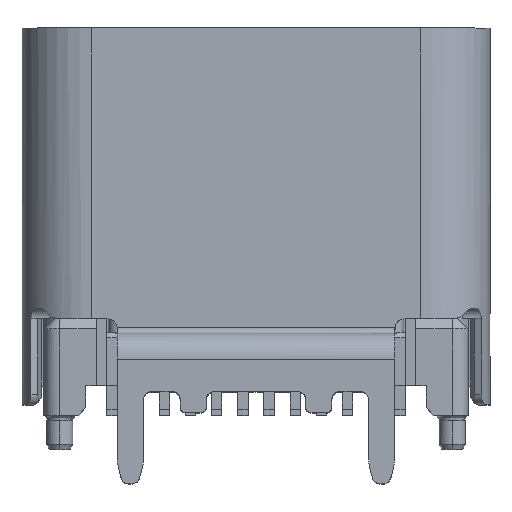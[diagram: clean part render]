
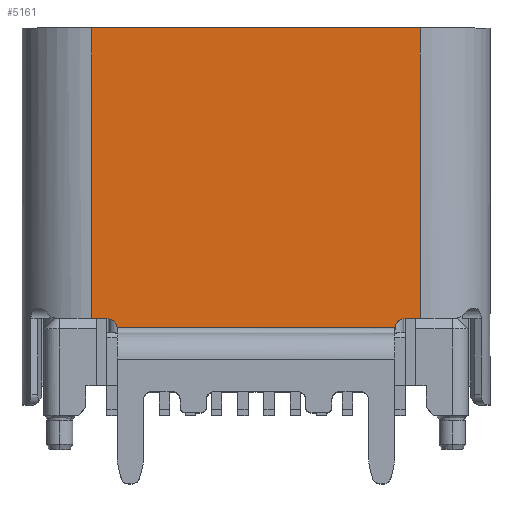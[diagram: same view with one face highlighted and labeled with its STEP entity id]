
A CAD part, top view. The second image highlights one B-rep face of the part: STEP entity #5161.
In plain terms, the highlighted face is planar.
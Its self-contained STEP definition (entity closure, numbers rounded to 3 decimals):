
#84 = EDGE_CURVE ( 'NONE', #32273, #32758, #39885, .T. ) ;
#189 = LINE ( 'NONE', #25824, #6939 ) ;
#207 = VERTEX_POINT ( 'NONE', #1972 ) ;
#1298 = DIRECTION ( 'NONE',  ( 0., 0., -1. ) ) ;
#1972 = CARTESIAN_POINT ( 'NONE',  ( 10.786, 16.807, 15.783 ) ) ;
#2573 = DIRECTION ( 'NONE',  ( 0., 0., -1. ) ) ;
#3392 = DIRECTION ( 'NONE',  ( 0., 1., 0. ) ) ;
#4640 = DIRECTION ( 'NONE',  ( -1., 0., 0. ) ) ;
#4763 = PLANE ( 'NONE',  #21060 ) ;
#5161 = ADVANCED_FACE ( 'NONE', ( #22440 ), #4763, .F. ) ;
#5346 = VECTOR ( 'NONE', #15647, 1000. ) ;
#5820 = LINE ( 'NONE', #41837, #13545 ) ;
#6440 = ORIENTED_EDGE ( 'NONE', *, *, #10337, .F. ) ;
#6939 = VECTOR ( 'NONE', #4640, 1000. ) ;
#7662 = CARTESIAN_POINT ( 'NONE',  ( 7.646, 11.257, 15.783 ) ) ;
#7954 = CARTESIAN_POINT ( 'NONE',  ( 10.786, 11.257, 15.783 ) ) ;
#8093 = LINE ( 'NONE', #14927, #35427 ) ;
#10337 = EDGE_CURVE ( 'NONE', #32758, #207, #46252, .T. ) ;
#10343 = DIRECTION ( 'NONE',  ( 1., 0., 0. ) ) ;
#10352 = CARTESIAN_POINT ( 'NONE',  ( 4.796, 17.007, 15.783 ) ) ;
#11971 = CIRCLE ( 'NONE', #33710, 0.2 ) ;
#12630 = VECTOR ( 'NONE', #3392, 1000. ) ;
#13208 = CARTESIAN_POINT ( 'NONE',  ( 4.796, 16.807, 15.783 ) ) ;
#13545 = VECTOR ( 'NONE', #37590, 1000. ) ;
#13662 = DIRECTION ( 'NONE',  ( -1., 0., 0. ) ) ;
#13855 = EDGE_CURVE ( 'NONE', #40624, #32273, #23616, .T. ) ;
#14927 = CARTESIAN_POINT ( 'NONE',  ( 7.646, 16.807, 15.783 ) ) ;
#15151 = EDGE_LOOP ( 'NONE', ( #35538, #16349, #26200, #38294, #6440, #44227, #28992, #37223 ) ) ;
#15647 = DIRECTION ( 'NONE',  ( 1., 0., 0. ) ) ;
#15738 = CARTESIAN_POINT ( 'NONE',  ( 4.995, 16.987, 15.783 ) ) ;
#16349 = ORIENTED_EDGE ( 'NONE', *, *, #31083, .F. ) ;
#18741 = EDGE_CURVE ( 'NONE', #30999, #23486, #20924, .T. ) ;
#19471 = EDGE_CURVE ( 'NONE', #39124, #39038, #11971, .T. ) ;
#20554 = DIRECTION ( 'NONE',  ( 0., -1., 0. ) ) ;
#20924 = CIRCLE ( 'NONE', #42729, 0.2 ) ;
#20998 = CARTESIAN_POINT ( 'NONE',  ( 4.506, 14.122, 15.783 ) ) ;
#21060 = AXIS2_PLACEMENT_3D ( 'NONE', #21969, #36304, #25468 ) ;
#21969 = CARTESIAN_POINT ( 'NONE',  ( 7.646, 14.122, 15.783 ) ) ;
#22440 = FACE_OUTER_BOUND ( 'NONE', #15151, .T. ) ;
#22619 = EDGE_CURVE ( 'NONE', #39038, #40624, #8093, .T. ) ;
#23486 = VERTEX_POINT ( 'NONE', #44346 ) ;
#23616 = LINE ( 'NONE', #20998, #45606 ) ;
#25164 = EDGE_CURVE ( 'NONE', #207, #30999, #5820, .T. ) ;
#25468 = DIRECTION ( 'NONE',  ( 1., 0., 0. ) ) ;
#25824 = CARTESIAN_POINT ( 'NONE',  ( 7.646, 16.987, 15.783 ) ) ;
#26200 = ORIENTED_EDGE ( 'NONE', *, *, #18741, .F. ) ;
#28992 = ORIENTED_EDGE ( 'NONE', *, *, #13855, .F. ) ;
#30999 = VERTEX_POINT ( 'NONE', #42562 ) ;
#31083 = EDGE_CURVE ( 'NONE', #23486, #39124, #189, .T. ) ;
#31361 = CARTESIAN_POINT ( 'NONE',  ( 10.786, 14.122, 15.783 ) ) ;
#32273 = VERTEX_POINT ( 'NONE', #45151 ) ;
#32758 = VERTEX_POINT ( 'NONE', #7954 ) ;
#32785 = DIRECTION ( 'NONE',  ( -1., 0., 0. ) ) ;
#33710 = AXIS2_PLACEMENT_3D ( 'NONE', #10352, #2573, #13662 ) ;
#35427 = VECTOR ( 'NONE', #32785, 1000. ) ;
#35494 = CARTESIAN_POINT ( 'NONE',  ( 10.496, 17.007, 15.783 ) ) ;
#35538 = ORIENTED_EDGE ( 'NONE', *, *, #19471, .F. ) ;
#36304 = DIRECTION ( 'NONE',  ( 0., 0., 1. ) ) ;
#37223 = ORIENTED_EDGE ( 'NONE', *, *, #22619, .F. ) ;
#37590 = DIRECTION ( 'NONE',  ( -1., 0., 0. ) ) ;
#38294 = ORIENTED_EDGE ( 'NONE', *, *, #25164, .F. ) ;
#39038 = VERTEX_POINT ( 'NONE', #13208 ) ;
#39124 = VERTEX_POINT ( 'NONE', #15738 ) ;
#39885 = LINE ( 'NONE', #7662, #5346 ) ;
#40624 = VERTEX_POINT ( 'NONE', #45576 ) ;
#41837 = CARTESIAN_POINT ( 'NONE',  ( 7.646, 16.807, 15.783 ) ) ;
#42562 = CARTESIAN_POINT ( 'NONE',  ( 10.496, 16.807, 15.783 ) ) ;
#42729 = AXIS2_PLACEMENT_3D ( 'NONE', #35494, #1298, #10343 ) ;
#44227 = ORIENTED_EDGE ( 'NONE', *, *, #84, .F. ) ;
#44346 = CARTESIAN_POINT ( 'NONE',  ( 10.297, 16.987, 15.783 ) ) ;
#45151 = CARTESIAN_POINT ( 'NONE',  ( 4.506, 11.257, 15.783 ) ) ;
#45576 = CARTESIAN_POINT ( 'NONE',  ( 4.506, 16.807, 15.783 ) ) ;
#45606 = VECTOR ( 'NONE', #20554, 1000. ) ;
#46252 = LINE ( 'NONE', #31361, #12630 ) ;
